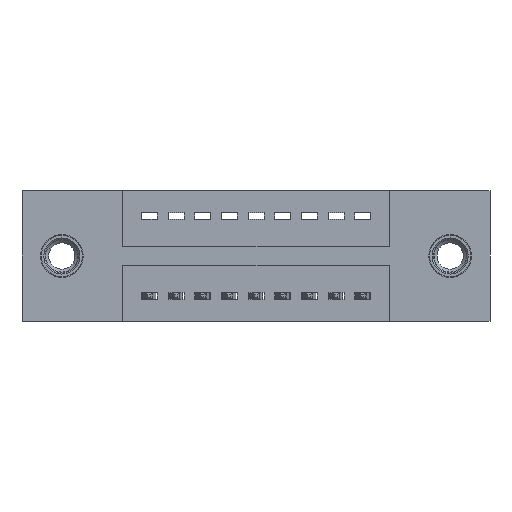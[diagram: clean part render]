
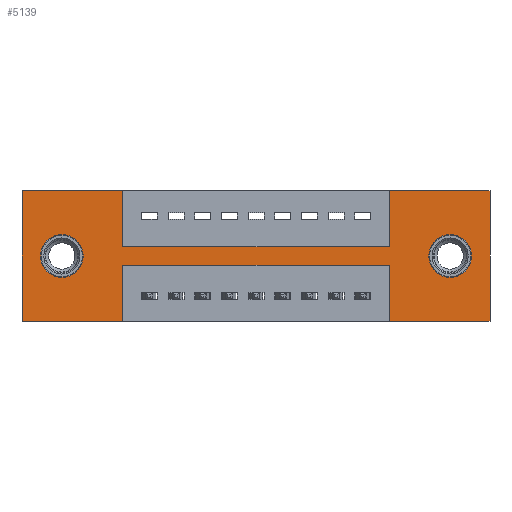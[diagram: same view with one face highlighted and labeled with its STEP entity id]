
A CAD part, front view. The second image highlights one B-rep face of the part: STEP entity #5139.
In plain terms, the highlighted planar face has unit normal (0, -1, 0).
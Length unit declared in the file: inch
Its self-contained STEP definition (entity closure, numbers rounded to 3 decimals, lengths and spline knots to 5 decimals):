
#54 = EDGE_CURVE ( 'NONE', #399, #1755, #4608, .T. ) ;
#65 = EDGE_CURVE ( 'NONE', #6787, #7938, #3822, .T. ) ;
#127 = ORIENTED_EDGE ( 'NONE', *, *, #4064, .F. ) ;
#128 = VECTOR ( 'NONE', #4551, 39.37008 ) ;
#198 = CARTESIAN_POINT ( 'NONE',  ( 1.3775, 0., -0.28 ) ) ;
#207 = CARTESIAN_POINT ( 'NONE',  ( 1.3775, 0., 0. ) ) ;
#270 = PLANE ( 'NONE',  #335 ) ;
#335 = AXIS2_PLACEMENT_3D ( 'NONE', #8648, #10419, #2653 ) ;
#399 = VERTEX_POINT ( 'NONE', #5984 ) ;
#612 = LINE ( 'NONE', #7901, #1678 ) ;
#624 = DIRECTION ( 'NONE',  ( 0., 0., 1. ) ) ;
#709 = DIRECTION ( 'NONE',  ( 0., 1., 0. ) ) ;
#823 = DIRECTION ( 'NONE',  ( 0., 0., -1. ) ) ;
#872 = CIRCLE ( 'NONE', #9947, 0.08 ) ;
#1045 = VERTEX_POINT ( 'NONE', #9443 ) ;
#1056 = DIRECTION ( 'NONE',  ( 0., 0., -1. ) ) ;
#1123 = EDGE_CURVE ( 'NONE', #2825, #10146, #612, .T. ) ;
#1196 = DIRECTION ( 'NONE',  ( 0., 0., 1. ) ) ;
#1238 = VECTOR ( 'NONE', #3574, 39.37008 ) ;
#1246 = CARTESIAN_POINT ( 'NONE',  ( 1.3775, 0., -0.21 ) ) ;
#1469 = VECTOR ( 'NONE', #8011, 39.37008 ) ;
#1473 = VECTOR ( 'NONE', #7880, 39.37008 ) ;
#1505 = FACE_BOUND ( 'NONE', #10991, .T. ) ;
#1543 = EDGE_LOOP ( 'NONE', ( #8981, #8024, #6076, #8925, #2368, #1681, #127, #10333, #7105, #9699, #4138, #4713 ) ) ;
#1678 = VECTOR ( 'NONE', #9516, 39.37008 ) ;
#1681 = ORIENTED_EDGE ( 'NONE', *, *, #8728, .F. ) ;
#1755 = VERTEX_POINT ( 'NONE', #10923 ) ;
#1874 = LINE ( 'NONE', #5687, #8666 ) ;
#1933 = EDGE_CURVE ( 'NONE', #7938, #399, #6017, .T. ) ;
#2368 = ORIENTED_EDGE ( 'NONE', *, *, #3098, .F. ) ;
#2555 = CARTESIAN_POINT ( 'NONE',  ( 0., 0., 0. ) ) ;
#2653 = DIRECTION ( 'NONE',  ( 0., 0., -1. ) ) ;
#2721 = CARTESIAN_POINT ( 'NONE',  ( 1.755, 0., 0. ) ) ;
#2798 = LINE ( 'NONE', #2555, #9064 ) ;
#2825 = VERTEX_POINT ( 'NONE', #198 ) ;
#2833 = VECTOR ( 'NONE', #1196, 39.37008 ) ;
#2915 = CARTESIAN_POINT ( 'NONE',  ( 0.3775, 0., 0. ) ) ;
#2979 = VECTOR ( 'NONE', #4327, 39.37008 ) ;
#2993 = VERTEX_POINT ( 'NONE', #7236 ) ;
#3098 = EDGE_CURVE ( 'NONE', #8940, #6310, #1874, .T. ) ;
#3135 = EDGE_CURVE ( 'NONE', #10226, #8115, #3203, .T. ) ;
#3146 = EDGE_CURVE ( 'NONE', #1755, #5092, #5182, .T. ) ;
#3202 = CARTESIAN_POINT ( 'NONE',  ( 0., 0., -0.49 ) ) ;
#3203 = CIRCLE ( 'NONE', #8683, 0.08 ) ;
#3478 = LINE ( 'NONE', #6089, #1238 ) ;
#3574 = DIRECTION ( 'NONE',  ( 1., 0., 0. ) ) ;
#3822 = LINE ( 'NONE', #1246, #1469 ) ;
#3962 = CARTESIAN_POINT ( 'NONE',  ( 0., 0., 0. ) ) ;
#4064 = EDGE_CURVE ( 'NONE', #10146, #7336, #6781, .T. ) ;
#4080 = DIRECTION ( 'NONE',  ( 0., 1., 0. ) ) ;
#4138 = ORIENTED_EDGE ( 'NONE', *, *, #54, .F. ) ;
#4327 = DIRECTION ( 'NONE',  ( 1., 0., 0. ) ) ;
#4381 = ORIENTED_EDGE ( 'NONE', *, *, #3135, .T. ) ;
#4551 = DIRECTION ( 'NONE',  ( 0., 0., -1. ) ) ;
#4608 = LINE ( 'NONE', #2721, #6876 ) ;
#4652 = LINE ( 'NONE', #8967, #128 ) ;
#4713 = ORIENTED_EDGE ( 'NONE', *, *, #1933, .F. ) ;
#4879 = CARTESIAN_POINT ( 'NONE',  ( 1.6055, 0., -0.245 ) ) ;
#4897 = EDGE_CURVE ( 'NONE', #6807, #2993, #6810, .T. ) ;
#5069 = CARTESIAN_POINT ( 'NONE',  ( 0., 0., 0. ) ) ;
#5092 = VERTEX_POINT ( 'NONE', #9391 ) ;
#5139 = ADVANCED_FACE ( 'NONE', ( #1505, #7757, #9722 ), #270, .T. ) ;
#5144 = CIRCLE ( 'NONE', #9521, 0.08 ) ;
#5182 = LINE ( 'NONE', #3202, #9452 ) ;
#5187 = EDGE_CURVE ( 'NONE', #1045, #6787, #3478, .T. ) ;
#5228 = ORIENTED_EDGE ( 'NONE', *, *, #7067, .T. ) ;
#5262 = CARTESIAN_POINT ( 'NONE',  ( 0.3775, 0., -0.49 ) ) ;
#5273 = ORIENTED_EDGE ( 'NONE', *, *, #9151, .T. ) ;
#5358 = VERTEX_POINT ( 'NONE', #2915 ) ;
#5375 = DIRECTION ( 'NONE',  ( 0., 0., 1. ) ) ;
#5687 = CARTESIAN_POINT ( 'NONE',  ( 0., 0., 0. ) ) ;
#5728 = DIRECTION ( 'NONE',  ( 0., 1., 0. ) ) ;
#5820 = DIRECTION ( 'NONE',  ( 0., 0., 1. ) ) ;
#5886 = EDGE_CURVE ( 'NONE', #6310, #5358, #2798, .T. ) ;
#5984 = CARTESIAN_POINT ( 'NONE',  ( 1.755, 0., 0. ) ) ;
#6017 = LINE ( 'NONE', #5069, #2979 ) ;
#6076 = ORIENTED_EDGE ( 'NONE', *, *, #10677, .F. ) ;
#6089 = CARTESIAN_POINT ( 'NONE',  ( 0.3775, 0., -0.21 ) ) ;
#6165 = CARTESIAN_POINT ( 'NONE',  ( 1.3775, 0., -0.21 ) ) ;
#6292 = LINE ( 'NONE', #8826, #2833 ) ;
#6305 = LINE ( 'NONE', #6469, #8592 ) ;
#6310 = VERTEX_POINT ( 'NONE', #3962 ) ;
#6367 = CARTESIAN_POINT ( 'NONE',  ( 0.1495, 0., -0.165 ) ) ;
#6469 = CARTESIAN_POINT ( 'NONE',  ( 0., 0., -0.49 ) ) ;
#6542 = CARTESIAN_POINT ( 'NONE',  ( 0.1495, 0., -0.325 ) ) ;
#6551 = EDGE_LOOP ( 'NONE', ( #5273, #4381 ) ) ;
#6781 = LINE ( 'NONE', #9526, #1473 ) ;
#6787 = VERTEX_POINT ( 'NONE', #6165 ) ;
#6807 = VERTEX_POINT ( 'NONE', #7825 ) ;
#6810 = CIRCLE ( 'NONE', #8386, 0.08 ) ;
#6876 = VECTOR ( 'NONE', #1056, 39.37008 ) ;
#7067 = EDGE_CURVE ( 'NONE', #2993, #6807, #5144, .T. ) ;
#7105 = ORIENTED_EDGE ( 'NONE', *, *, #9133, .F. ) ;
#7236 = CARTESIAN_POINT ( 'NONE',  ( 1.6055, 0., -0.325 ) ) ;
#7336 = VERTEX_POINT ( 'NONE', #5262 ) ;
#7494 = DIRECTION ( 'NONE',  ( -1., 0., 0. ) ) ;
#7757 = FACE_BOUND ( 'NONE', #6551, .T. ) ;
#7825 = CARTESIAN_POINT ( 'NONE',  ( 1.6055, 0., -0.165 ) ) ;
#7880 = DIRECTION ( 'NONE',  ( 0., 0., -1. ) ) ;
#7901 = CARTESIAN_POINT ( 'NONE',  ( 0.3775, 0., -0.28 ) ) ;
#7938 = VERTEX_POINT ( 'NONE', #207 ) ;
#8010 = DIRECTION ( 'NONE',  ( 0., 1., 0. ) ) ;
#8011 = DIRECTION ( 'NONE',  ( 0., 0., 1. ) ) ;
#8024 = ORIENTED_EDGE ( 'NONE', *, *, #5187, .F. ) ;
#8115 = VERTEX_POINT ( 'NONE', #6367 ) ;
#8373 = DIRECTION ( 'NONE',  ( 0., 0., -1. ) ) ;
#8386 = AXIS2_PLACEMENT_3D ( 'NONE', #4879, #709, #823 ) ;
#8416 = CARTESIAN_POINT ( 'NONE',  ( 1.6055, 0., -0.245 ) ) ;
#8515 = DIRECTION ( 'NONE',  ( 1., 0., 0. ) ) ;
#8592 = VECTOR ( 'NONE', #10719, 39.37008 ) ;
#8648 = CARTESIAN_POINT ( 'NONE',  ( 0., 0., -0.49 ) ) ;
#8666 = VECTOR ( 'NONE', #624, 39.37008 ) ;
#8683 = AXIS2_PLACEMENT_3D ( 'NONE', #10853, #5728, #5820 ) ;
#8728 = EDGE_CURVE ( 'NONE', #7336, #8940, #6305, .T. ) ;
#8826 = CARTESIAN_POINT ( 'NONE',  ( 1.3775, 0., -0.28 ) ) ;
#8925 = ORIENTED_EDGE ( 'NONE', *, *, #5886, .F. ) ;
#8940 = VERTEX_POINT ( 'NONE', #10039 ) ;
#8967 = CARTESIAN_POINT ( 'NONE',  ( 0.3775, 0., -0.21 ) ) ;
#8981 = ORIENTED_EDGE ( 'NONE', *, *, #65, .F. ) ;
#9064 = VECTOR ( 'NONE', #8515, 39.37008 ) ;
#9133 = EDGE_CURVE ( 'NONE', #5092, #2825, #6292, .T. ) ;
#9151 = EDGE_CURVE ( 'NONE', #8115, #10226, #872, .T. ) ;
#9391 = CARTESIAN_POINT ( 'NONE',  ( 1.3775, 0., -0.49 ) ) ;
#9443 = CARTESIAN_POINT ( 'NONE',  ( 0.3775, 0., -0.21 ) ) ;
#9452 = VECTOR ( 'NONE', #7494, 39.37008 ) ;
#9499 = ORIENTED_EDGE ( 'NONE', *, *, #4897, .T. ) ;
#9516 = DIRECTION ( 'NONE',  ( -1., 0., 0. ) ) ;
#9521 = AXIS2_PLACEMENT_3D ( 'NONE', #8416, #4080, #8373 ) ;
#9526 = CARTESIAN_POINT ( 'NONE',  ( 0.3775, 0., -0.28 ) ) ;
#9608 = CARTESIAN_POINT ( 'NONE',  ( 0.1495, 0., -0.245 ) ) ;
#9699 = ORIENTED_EDGE ( 'NONE', *, *, #3146, .F. ) ;
#9722 = FACE_OUTER_BOUND ( 'NONE', #1543, .T. ) ;
#9947 = AXIS2_PLACEMENT_3D ( 'NONE', #9608, #8010, #5375 ) ;
#10039 = CARTESIAN_POINT ( 'NONE',  ( 0., 0., -0.49 ) ) ;
#10146 = VERTEX_POINT ( 'NONE', #10605 ) ;
#10226 = VERTEX_POINT ( 'NONE', #6542 ) ;
#10333 = ORIENTED_EDGE ( 'NONE', *, *, #1123, .F. ) ;
#10419 = DIRECTION ( 'NONE',  ( 0., -1., 0. ) ) ;
#10605 = CARTESIAN_POINT ( 'NONE',  ( 0.3775, 0., -0.28 ) ) ;
#10677 = EDGE_CURVE ( 'NONE', #5358, #1045, #4652, .T. ) ;
#10719 = DIRECTION ( 'NONE',  ( -1., 0., 0. ) ) ;
#10853 = CARTESIAN_POINT ( 'NONE',  ( 0.1495, 0., -0.245 ) ) ;
#10923 = CARTESIAN_POINT ( 'NONE',  ( 1.755, 0., -0.49 ) ) ;
#10991 = EDGE_LOOP ( 'NONE', ( #9499, #5228 ) ) ;
